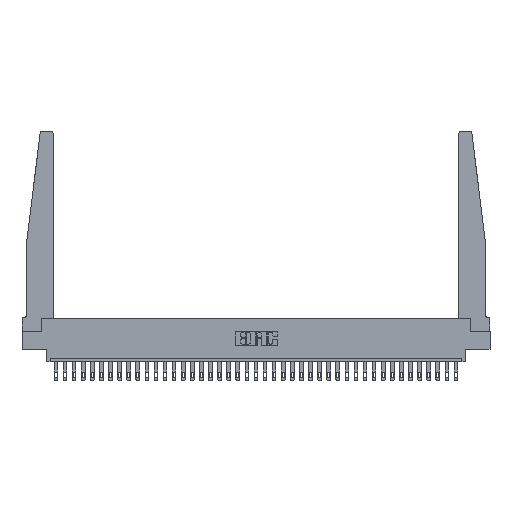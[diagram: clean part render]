
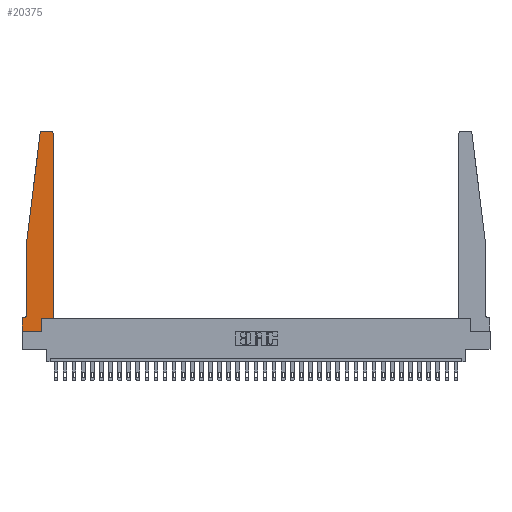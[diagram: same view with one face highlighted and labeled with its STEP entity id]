
A CAD part, top view. The second image highlights one B-rep face of the part: STEP entity #20375.
In plain terms, the highlighted planar face has unit normal (0, 0, 1).
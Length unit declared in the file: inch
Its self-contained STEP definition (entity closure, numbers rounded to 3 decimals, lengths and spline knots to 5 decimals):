
#620 = ORIENTED_EDGE ( 'NONE', *, *, #28909, .T. ) ;
#977 = ORIENTED_EDGE ( 'NONE', *, *, #13829, .T. ) ;
#1401 = LINE ( 'NONE', #19277, #3327 ) ;
#1478 = CARTESIAN_POINT ( 'NONE',  ( 0.425, 0.18, 0.37 ) ) ;
#1780 = DIRECTION ( 'NONE',  ( 0., -1., 0. ) ) ;
#1799 = CIRCLE ( 'NONE', #32519, 0.03 ) ;
#1850 = EDGE_CURVE ( 'NONE', #19716, #9011, #10823, .T. ) ;
#1984 = VECTOR ( 'NONE', #29069, 39.37008 ) ;
#2434 = ORIENTED_EDGE ( 'NONE', *, *, #7708, .T. ) ;
#3081 = VERTEX_POINT ( 'NONE', #30976 ) ;
#3141 = CARTESIAN_POINT ( 'NONE',  ( 0.24675, 2.72367, 0.37 ) ) ;
#3327 = VECTOR ( 'NONE', #26766, 39.37008 ) ;
#3605 = ORIENTED_EDGE ( 'NONE', *, *, #30286, .T. ) ;
#3712 = VECTOR ( 'NONE', #8565, 39.37008 ) ;
#4573 = VERTEX_POINT ( 'NONE', #28598 ) ;
#4964 = ORIENTED_EDGE ( 'NONE', *, *, #31257, .T. ) ;
#5623 = ORIENTED_EDGE ( 'NONE', *, *, #22750, .T. ) ;
#6266 = LINE ( 'NONE', #26334, #3712 ) ;
#6424 = VECTOR ( 'NONE', #1780, 39.37008 ) ;
#6696 = AXIS2_PLACEMENT_3D ( 'NONE', #14265, #29719, #27060 ) ;
#6830 = EDGE_CURVE ( 'NONE', #9991, #3081, #9711, .T. ) ;
#7708 = EDGE_CURVE ( 'NONE', #3081, #4573, #13950, .T. ) ;
#7924 = EDGE_CURVE ( 'NONE', #4573, #15946, #30066, .T. ) ;
#8329 = CARTESIAN_POINT ( 'NONE',  ( 0.065, 1.25, 0.37 ) ) ;
#8565 = DIRECTION ( 'NONE',  ( -0.122, -0.992, 0. ) ) ;
#8799 = ORIENTED_EDGE ( 'NONE', *, *, #18671, .T. ) ;
#9011 = VERTEX_POINT ( 'NONE', #32146 ) ;
#9108 = CARTESIAN_POINT ( 'NONE',  ( 0.425, 0.18, 0.37 ) ) ;
#9340 = VERTEX_POINT ( 'NONE', #26165 ) ;
#9711 = LINE ( 'NONE', #1478, #10700 ) ;
#9991 = VERTEX_POINT ( 'NONE', #21208 ) ;
#10202 = DIRECTION ( 'NONE',  ( 0., -1., 0. ) ) ;
#10700 = VECTOR ( 'NONE', #11743, 39.37008 ) ;
#10823 = LINE ( 'NONE', #8329, #29067 ) ;
#10893 = DIRECTION ( 'NONE',  ( -1., 0., 0. ) ) ;
#11453 = FACE_OUTER_BOUND ( 'NONE', #23097, .T. ) ;
#11743 = DIRECTION ( 'NONE',  ( 1., 0., 0. ) ) ;
#11828 = VECTOR ( 'NONE', #13285, 39.37008 ) ;
#12731 = DIRECTION ( 'NONE',  ( 0., 0., 1. ) ) ;
#13285 = DIRECTION ( 'NONE',  ( 1., 0., 0. ) ) ;
#13320 = VERTEX_POINT ( 'NONE', #25008 ) ;
#13370 = VECTOR ( 'NONE', #10893, 39.37008 ) ;
#13829 = EDGE_CURVE ( 'NONE', #16541, #15767, #17009, .T. ) ;
#13950 = LINE ( 'NONE', #9108, #1984 ) ;
#13995 = DIRECTION ( 'NONE',  ( 1., 0., 0. ) ) ;
#14265 = CARTESIAN_POINT ( 'NONE',  ( 0., 0.1875, 0.37 ) ) ;
#14377 = CARTESIAN_POINT ( 'NONE',  ( 0., 0.1875, 0.37 ) ) ;
#15767 = VERTEX_POINT ( 'NONE', #23918 ) ;
#15946 = VERTEX_POINT ( 'NONE', #21688 ) ;
#16541 = VERTEX_POINT ( 'NONE', #14377 ) ;
#17009 = LINE ( 'NONE', #24968, #6424 ) ;
#17793 = VERTEX_POINT ( 'NONE', #3141 ) ;
#17931 = LINE ( 'NONE', #28398, #11828 ) ;
#18341 = CARTESIAN_POINT ( 'NONE',  ( 0.395, 2.72, 0.37 ) ) ;
#18671 = EDGE_CURVE ( 'NONE', #9340, #17793, #1799, .T. ) ;
#19035 = CARTESIAN_POINT ( 'NONE',  ( 0.25, 2.75, 0.37 ) ) ;
#19189 = ORIENTED_EDGE ( 'NONE', *, *, #6830, .T. ) ;
#19277 = CARTESIAN_POINT ( 'NONE',  ( 0.065, 0.1875, 0.37 ) ) ;
#19438 = ORIENTED_EDGE ( 'NONE', *, *, #1850, .T. ) ;
#19716 = VERTEX_POINT ( 'NONE', #22964 ) ;
#20375 = ADVANCED_FACE ( 'NONE', ( #11453 ), #21726, .T. ) ;
#20690 = EDGE_CURVE ( 'NONE', #9011, #28274, #32139, .T. ) ;
#21208 = CARTESIAN_POINT ( 'NONE',  ( 0.2605, 0.18, 0.37 ) ) ;
#21447 = DIRECTION ( 'NONE',  ( 0., 0., 1. ) ) ;
#21559 = ORIENTED_EDGE ( 'NONE', *, *, #7924, .T. ) ;
#21688 = CARTESIAN_POINT ( 'NONE',  ( 0.395, 2.75, 0.37 ) ) ;
#21726 = PLANE ( 'NONE',  #6696 ) ;
#22750 = EDGE_CURVE ( 'NONE', #13320, #9991, #24433, .T. ) ;
#22964 = CARTESIAN_POINT ( 'NONE',  ( 0.065, 1.25, 0.37 ) ) ;
#23097 = EDGE_LOOP ( 'NONE', ( #620, #8799, #28955, #19438, #23873, #4964, #977, #3605, #5623, #19189, #2434, #21559 ) ) ;
#23675 = DIRECTION ( 'NONE',  ( 0., 0., -1. ) ) ;
#23730 = VECTOR ( 'NONE', #31590, 39.37008 ) ;
#23873 = ORIENTED_EDGE ( 'NONE', *, *, #20690, .T. ) ;
#23918 = CARTESIAN_POINT ( 'NONE',  ( 0., 0., 0.37 ) ) ;
#23943 = CARTESIAN_POINT ( 'NONE',  ( 0.2605, 0.18, 0.37 ) ) ;
#24433 = LINE ( 'NONE', #23943, #23730 ) ;
#24968 = CARTESIAN_POINT ( 'NONE',  ( 0., 0., 0.37 ) ) ;
#25008 = CARTESIAN_POINT ( 'NONE',  ( 0.2605, 0., 0.37 ) ) ;
#25860 = DIRECTION ( 'NONE',  ( -1., 0., 0. ) ) ;
#26165 = CARTESIAN_POINT ( 'NONE',  ( 0.27653, 2.75, 0.37 ) ) ;
#26270 = EDGE_CURVE ( 'NONE', #17793, #19716, #6266, .T. ) ;
#26334 = CARTESIAN_POINT ( 'NONE',  ( 0.065, 1.25, 0.37 ) ) ;
#26467 = CARTESIAN_POINT ( 'NONE',  ( 0.015, 0.1875, 0.37 ) ) ;
#26766 = DIRECTION ( 'NONE',  ( -1., 0., 0. ) ) ;
#26935 = CARTESIAN_POINT ( 'NONE',  ( 0.27653, 2.72, 0.37 ) ) ;
#27060 = DIRECTION ( 'NONE',  ( 1., 0., 0. ) ) ;
#27361 = AXIS2_PLACEMENT_3D ( 'NONE', #28694, #23675, #25860 ) ;
#28274 = VERTEX_POINT ( 'NONE', #26467 ) ;
#28398 = CARTESIAN_POINT ( 'NONE',  ( 0., 0., 0.37 ) ) ;
#28479 = DIRECTION ( 'NONE',  ( 1., 0., 0. ) ) ;
#28598 = CARTESIAN_POINT ( 'NONE',  ( 0.425, 2.72, 0.37 ) ) ;
#28694 = CARTESIAN_POINT ( 'NONE',  ( 0.015, 0.2375, 0.37 ) ) ;
#28909 = EDGE_CURVE ( 'NONE', #15946, #9340, #30672, .T. ) ;
#28955 = ORIENTED_EDGE ( 'NONE', *, *, #26270, .T. ) ;
#29067 = VECTOR ( 'NONE', #10202, 39.37008 ) ;
#29069 = DIRECTION ( 'NONE',  ( 0., 1., 0. ) ) ;
#29719 = DIRECTION ( 'NONE',  ( 0., 0., 1. ) ) ;
#30066 = CIRCLE ( 'NONE', #31653, 0.03 ) ;
#30286 = EDGE_CURVE ( 'NONE', #15767, #13320, #17931, .T. ) ;
#30672 = LINE ( 'NONE', #19035, #13370 ) ;
#30976 = CARTESIAN_POINT ( 'NONE',  ( 0.425, 0.18, 0.37 ) ) ;
#31257 = EDGE_CURVE ( 'NONE', #28274, #16541, #1401, .T. ) ;
#31590 = DIRECTION ( 'NONE',  ( 0., 1., 0. ) ) ;
#31653 = AXIS2_PLACEMENT_3D ( 'NONE', #18341, #12731, #28479 ) ;
#32139 = CIRCLE ( 'NONE', #27361, 0.05 ) ;
#32146 = CARTESIAN_POINT ( 'NONE',  ( 0.065, 0.2375, 0.37 ) ) ;
#32519 = AXIS2_PLACEMENT_3D ( 'NONE', #26935, #21447, #13995 ) ;
